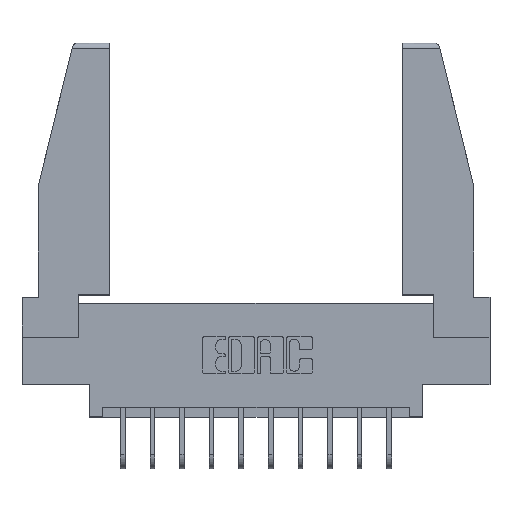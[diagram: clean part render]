
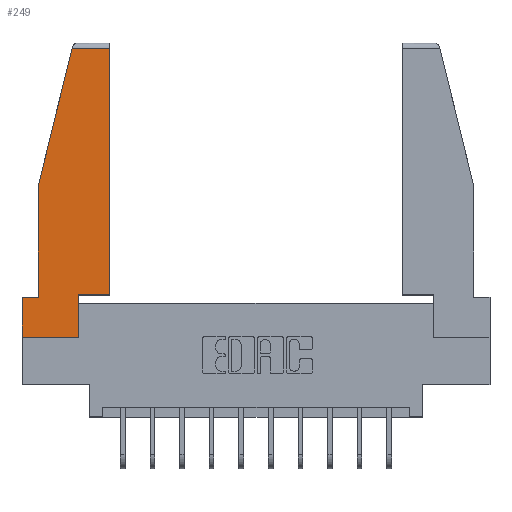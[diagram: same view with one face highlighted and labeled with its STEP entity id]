
A CAD part, top view. The second image highlights one B-rep face of the part: STEP entity #249.
In plain terms, the highlighted planar face has unit normal (0, 0, 1).
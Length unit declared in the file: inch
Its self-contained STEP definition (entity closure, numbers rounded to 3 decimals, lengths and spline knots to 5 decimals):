
#22 = VECTOR ( 'NONE', #14565, 39.37008 ) ;
#114 = DIRECTION ( 'NONE',  ( -1., 0., 0. ) ) ;
#150 = LINE ( 'NONE', #13981, #8453 ) ;
#249 = ADVANCED_FACE ( 'NONE', ( #10222 ), #6305, .T. ) ;
#897 = LINE ( 'NONE', #6487, #1483 ) ;
#1483 = VECTOR ( 'NONE', #15294, 39.37008 ) ;
#1577 = CARTESIAN_POINT ( 'NONE',  ( 0.2636, 1.52, 0. ) ) ;
#1594 = LINE ( 'NONE', #4634, #9711 ) ;
#1608 = LINE ( 'NONE', #9246, #8729 ) ;
#2216 = CARTESIAN_POINT ( 'NONE',  ( 0.297, 0., 0. ) ) ;
#2345 = VERTEX_POINT ( 'NONE', #11686 ) ;
#2435 = CARTESIAN_POINT ( 'NONE',  ( 0., 0., 0. ) ) ;
#2524 = CARTESIAN_POINT ( 'NONE',  ( 0.271, 1.55, 0. ) ) ;
#2595 = CARTESIAN_POINT ( 'NONE',  ( 0.297, 0., 0. ) ) ;
#2747 = ORIENTED_EDGE ( 'NONE', *, *, #7016, .T. ) ;
#2822 = CARTESIAN_POINT ( 'NONE',  ( 0.461, 1.52, 0. ) ) ;
#3374 = ORIENTED_EDGE ( 'NONE', *, *, #4504, .T. ) ;
#3637 = EDGE_CURVE ( 'NONE', #7140, #11415, #1608, .T. ) ;
#3697 = CARTESIAN_POINT ( 'NONE',  ( 0., 0., 0. ) ) ;
#3756 = DIRECTION ( 'NONE',  ( 1., 0., 0. ) ) ;
#4165 = CARTESIAN_POINT ( 'NONE',  ( 0.297, 0.223, 0. ) ) ;
#4170 = ORIENTED_EDGE ( 'NONE', *, *, #11633, .T. ) ;
#4203 = DIRECTION ( 'NONE',  ( -1., 0., 0. ) ) ;
#4504 = EDGE_CURVE ( 'NONE', #9888, #7937, #14953, .T. ) ;
#4634 = CARTESIAN_POINT ( 'NONE',  ( 0.086, 0.8, 0. ) ) ;
#4635 = VERTEX_POINT ( 'NONE', #2435 ) ;
#5095 = VECTOR ( 'NONE', #15225, 39.37008 ) ;
#5272 = CARTESIAN_POINT ( 'NONE',  ( 0.461, 0.223, 0. ) ) ;
#5321 = CARTESIAN_POINT ( 'NONE',  ( 0., 0., 0. ) ) ;
#5400 = CARTESIAN_POINT ( 'NONE',  ( 0., 1.52, 0. ) ) ;
#6042 = EDGE_CURVE ( 'NONE', #10852, #14263, #150, .T. ) ;
#6305 = PLANE ( 'NONE',  #8108 ) ;
#6487 = CARTESIAN_POINT ( 'NONE',  ( 0.297, 0.223, 0. ) ) ;
#6775 = DIRECTION ( 'NONE',  ( 0., -1., 0. ) ) ;
#6950 = LINE ( 'NONE', #14275, #13079 ) ;
#7016 = EDGE_CURVE ( 'NONE', #7937, #10852, #897, .T. ) ;
#7140 = VERTEX_POINT ( 'NONE', #7404 ) ;
#7404 = CARTESIAN_POINT ( 'NONE',  ( 0.086, 0.21, 0. ) ) ;
#7710 = ORIENTED_EDGE ( 'NONE', *, *, #12249, .T. ) ;
#7937 = VERTEX_POINT ( 'NONE', #4165 ) ;
#8108 = AXIS2_PLACEMENT_3D ( 'NONE', #3697, #12615, #3756 ) ;
#8119 = ORIENTED_EDGE ( 'NONE', *, *, #6042, .T. ) ;
#8453 = VECTOR ( 'NONE', #9101, 39.37008 ) ;
#8455 = DIRECTION ( 'NONE',  ( 0., -1., 0. ) ) ;
#8729 = VECTOR ( 'NONE', #4203, 39.37008 ) ;
#9101 = DIRECTION ( 'NONE',  ( 0., 1., 0. ) ) ;
#9246 = CARTESIAN_POINT ( 'NONE',  ( 0., 0.21, 0. ) ) ;
#9288 = LINE ( 'NONE', #5321, #14184 ) ;
#9475 = VECTOR ( 'NONE', #114, 39.37008 ) ;
#9623 = ORIENTED_EDGE ( 'NONE', *, *, #12796, .T. ) ;
#9711 = VECTOR ( 'NONE', #8455, 39.37008 ) ;
#9812 = CARTESIAN_POINT ( 'NONE',  ( 0., 0.21, 0. ) ) ;
#9888 = VERTEX_POINT ( 'NONE', #2595 ) ;
#10048 = EDGE_CURVE ( 'NONE', #11415, #4635, #6950, .T. ) ;
#10222 = FACE_OUTER_BOUND ( 'NONE', #11372, .T. ) ;
#10436 = LINE ( 'NONE', #5400, #9475 ) ;
#10852 = VERTEX_POINT ( 'NONE', #5272 ) ;
#11372 = EDGE_LOOP ( 'NONE', ( #8119, #7710, #9623, #14468, #14734, #12892, #4170, #3374, #2747 ) ) ;
#11415 = VERTEX_POINT ( 'NONE', #9812 ) ;
#11633 = EDGE_CURVE ( 'NONE', #4635, #9888, #9288, .T. ) ;
#11686 = CARTESIAN_POINT ( 'NONE',  ( 0.086, 0.8, 0. ) ) ;
#12249 = EDGE_CURVE ( 'NONE', #14263, #12290, #10436, .T. ) ;
#12290 = VERTEX_POINT ( 'NONE', #1577 ) ;
#12615 = DIRECTION ( 'NONE',  ( 0., 0., 1. ) ) ;
#12796 = EDGE_CURVE ( 'NONE', #12290, #2345, #15898, .T. ) ;
#12892 = ORIENTED_EDGE ( 'NONE', *, *, #10048, .T. ) ;
#13079 = VECTOR ( 'NONE', #6775, 39.37008 ) ;
#13981 = CARTESIAN_POINT ( 'NONE',  ( 0.461, 0.223, 0. ) ) ;
#14184 = VECTOR ( 'NONE', #15413, 39.37008 ) ;
#14263 = VERTEX_POINT ( 'NONE', #2822 ) ;
#14275 = CARTESIAN_POINT ( 'NONE',  ( 0., 0.21, 0. ) ) ;
#14468 = ORIENTED_EDGE ( 'NONE', *, *, #14987, .T. ) ;
#14565 = DIRECTION ( 'NONE',  ( 0., 1., 0. ) ) ;
#14734 = ORIENTED_EDGE ( 'NONE', *, *, #3637, .T. ) ;
#14953 = LINE ( 'NONE', #2216, #22 ) ;
#14987 = EDGE_CURVE ( 'NONE', #2345, #7140, #1594, .T. ) ;
#15225 = DIRECTION ( 'NONE',  ( -0.239, -0.971, 0. ) ) ;
#15294 = DIRECTION ( 'NONE',  ( 1., 0., 0. ) ) ;
#15413 = DIRECTION ( 'NONE',  ( 1., 0., 0. ) ) ;
#15898 = LINE ( 'NONE', #2524, #5095 ) ;
